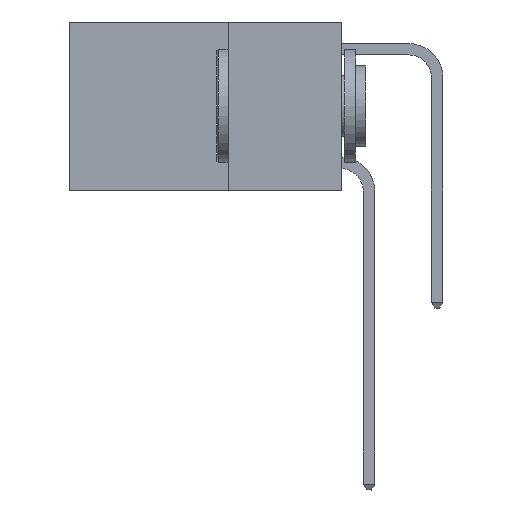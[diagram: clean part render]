
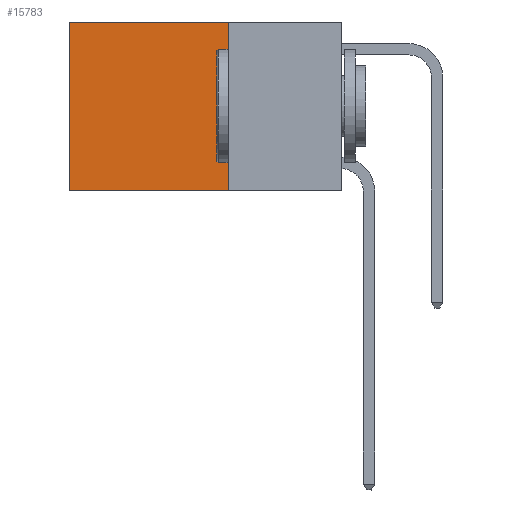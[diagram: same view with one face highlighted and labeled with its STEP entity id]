
A CAD part, left-side view. The second image highlights one B-rep face of the part: STEP entity #15783.
In plain terms, the highlighted planar face has unit normal (-1, 0, 0).
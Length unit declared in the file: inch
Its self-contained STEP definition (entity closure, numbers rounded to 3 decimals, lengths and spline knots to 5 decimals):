
#34 = AXIS2_PLACEMENT_3D ( 'NONE', #2191, #10482, #4021 ) ;
#1095 = VERTEX_POINT ( 'NONE', #13965 ) ;
#1341 = DIRECTION ( 'NONE',  ( 0., 0., -1. ) ) ;
#2191 = CARTESIAN_POINT ( 'NONE',  ( 0.2625, 0.25, 0. ) ) ;
#3948 = VECTOR ( 'NONE', #19049, 39.37008 ) ;
#4021 = DIRECTION ( 'NONE',  ( 0., 0., -1. ) ) ;
#5438 = CARTESIAN_POINT ( 'NONE',  ( 0.2625, 0.25, -0.37 ) ) ;
#5746 = VERTEX_POINT ( 'NONE', #11542 ) ;
#6423 = ORIENTED_EDGE ( 'NONE', *, *, #19396, .T. ) ;
#6830 = LINE ( 'NONE', #15107, #16761 ) ;
#7830 = CARTESIAN_POINT ( 'NONE',  ( 0.2625, 0.25, 0. ) ) ;
#7909 = ORIENTED_EDGE ( 'NONE', *, *, #9476, .T. ) ;
#9180 = EDGE_CURVE ( 'NONE', #19130, #19075, #14703, .T. ) ;
#9476 = EDGE_CURVE ( 'NONE', #1095, #5746, #27284, .T. ) ;
#10482 = DIRECTION ( 'NONE',  ( 1., 0., 0. ) ) ;
#10558 = DIRECTION ( 'NONE',  ( 0., 1., 0. ) ) ;
#10592 = EDGE_CURVE ( 'NONE', #19075, #5746, #23285, .T. ) ;
#11138 = VECTOR ( 'NONE', #10558, 39.37008 ) ;
#11542 = CARTESIAN_POINT ( 'NONE',  ( 0.2625, 0.6, -0.37 ) ) ;
#12519 = CARTESIAN_POINT ( 'NONE',  ( 0.2625, 0.25, -0.37 ) ) ;
#13061 = ORIENTED_EDGE ( 'NONE', *, *, #10592, .F. ) ;
#13965 = CARTESIAN_POINT ( 'NONE',  ( 0.2625, 0.6, 0. ) ) ;
#13996 = CARTESIAN_POINT ( 'NONE',  ( 0.2625, 0.6, 0. ) ) ;
#14703 = LINE ( 'NONE', #19476, #3948 ) ;
#15107 = CARTESIAN_POINT ( 'NONE',  ( 0.2625, 0.25, 0. ) ) ;
#15599 = EDGE_LOOP ( 'NONE', ( #7909, #13061, #17341, #6423 ) ) ;
#15783 = ADVANCED_FACE ( 'NONE', ( #19150 ), #24618, .F. ) ;
#16433 = VECTOR ( 'NONE', #1341, 39.37008 ) ;
#16761 = VECTOR ( 'NONE', #25737, 39.37008 ) ;
#17341 = ORIENTED_EDGE ( 'NONE', *, *, #9180, .F. ) ;
#19049 = DIRECTION ( 'NONE',  ( 0., 0., -1. ) ) ;
#19075 = VERTEX_POINT ( 'NONE', #5438 ) ;
#19130 = VERTEX_POINT ( 'NONE', #7830 ) ;
#19150 = FACE_OUTER_BOUND ( 'NONE', #15599, .T. ) ;
#19396 = EDGE_CURVE ( 'NONE', #19130, #1095, #6830, .T. ) ;
#19476 = CARTESIAN_POINT ( 'NONE',  ( 0.2625, 0.25, 0. ) ) ;
#23285 = LINE ( 'NONE', #12519, #11138 ) ;
#24618 = PLANE ( 'NONE',  #34 ) ;
#25737 = DIRECTION ( 'NONE',  ( 0., 1., 0. ) ) ;
#27284 = LINE ( 'NONE', #13996, #16433 ) ;
